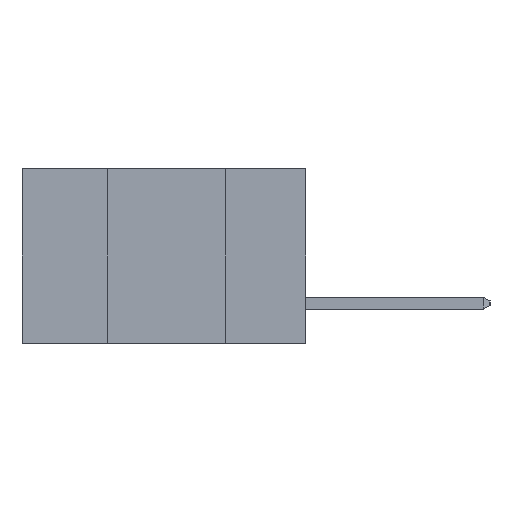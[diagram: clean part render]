
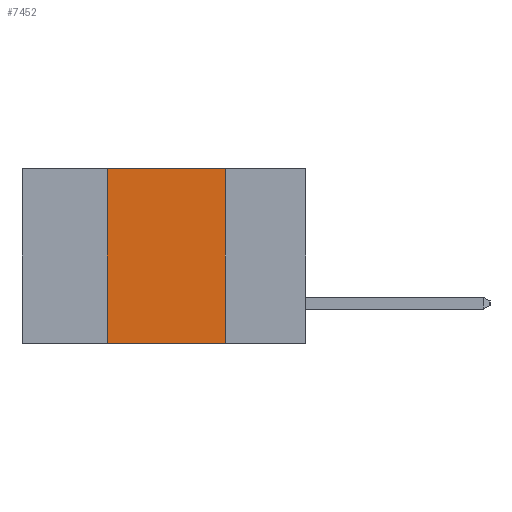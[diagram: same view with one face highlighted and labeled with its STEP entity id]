
A CAD part, left-side view. The second image highlights one B-rep face of the part: STEP entity #7452.
In plain terms, the highlighted planar face has unit normal (-1, 0, 0).
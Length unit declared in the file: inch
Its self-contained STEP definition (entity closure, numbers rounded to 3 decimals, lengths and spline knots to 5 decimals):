
#496 = DIRECTION ( 'NONE',  ( 0., 0., -1. ) ) ;
#1175 = DIRECTION ( 'NONE',  ( 0., -1., 0. ) ) ;
#1188 = DIRECTION ( 'NONE',  ( 0., 0., -1. ) ) ;
#1237 = CARTESIAN_POINT ( 'NONE',  ( 0., 0.6, -0.37 ) ) ;
#3038 = CARTESIAN_POINT ( 'NONE',  ( 0., 0.42, -0.37 ) ) ;
#3181 = ORIENTED_EDGE ( 'NONE', *, *, #9438, .F. ) ;
#3451 = CARTESIAN_POINT ( 'NONE',  ( 0., 0.6, 0. ) ) ;
#3650 = ORIENTED_EDGE ( 'NONE', *, *, #17198, .F. ) ;
#3734 = VERTEX_POINT ( 'NONE', #3038 ) ;
#5111 = FACE_OUTER_BOUND ( 'NONE', #14086, .T. ) ;
#5157 = CARTESIAN_POINT ( 'NONE',  ( 0., 0.17, 0. ) ) ;
#6205 = AXIS2_PLACEMENT_3D ( 'NONE', #3451, #9294, #496 ) ;
#6636 = ORIENTED_EDGE ( 'NONE', *, *, #11870, .F. ) ;
#6699 = EDGE_CURVE ( 'NONE', #3734, #7310, #6720, .T. ) ;
#6720 = LINE ( 'NONE', #1237, #14113 ) ;
#7310 = VERTEX_POINT ( 'NONE', #13053 ) ;
#7452 = ADVANCED_FACE ( 'NONE', ( #5111 ), #17558, .F. ) ;
#7536 = VERTEX_POINT ( 'NONE', #5157 ) ;
#9285 = CARTESIAN_POINT ( 'NONE',  ( 0., 0.42, 0. ) ) ;
#9288 = VECTOR ( 'NONE', #15101, 39.37008 ) ;
#9294 = DIRECTION ( 'NONE',  ( 1., 0., 0. ) ) ;
#9438 = EDGE_CURVE ( 'NONE', #12308, #7536, #16642, .T. ) ;
#9927 = CARTESIAN_POINT ( 'NONE',  ( 0., 0.17, 0. ) ) ;
#11161 = VECTOR ( 'NONE', #16178, 39.37008 ) ;
#11266 = ORIENTED_EDGE ( 'NONE', *, *, #6699, .T. ) ;
#11870 = EDGE_CURVE ( 'NONE', #7536, #7310, #12858, .T. ) ;
#12308 = VERTEX_POINT ( 'NONE', #17782 ) ;
#12858 = LINE ( 'NONE', #9927, #16156 ) ;
#13053 = CARTESIAN_POINT ( 'NONE',  ( 0., 0.17, -0.37 ) ) ;
#13679 = CARTESIAN_POINT ( 'NONE',  ( 0., 0.6, 0. ) ) ;
#14086 = EDGE_LOOP ( 'NONE', ( #6636, #3181, #3650, #11266 ) ) ;
#14113 = VECTOR ( 'NONE', #1175, 39.37008 ) ;
#14811 = LINE ( 'NONE', #9285, #11161 ) ;
#15101 = DIRECTION ( 'NONE',  ( 0., -1., 0. ) ) ;
#16156 = VECTOR ( 'NONE', #1188, 39.37008 ) ;
#16178 = DIRECTION ( 'NONE',  ( 0., 0., 1. ) ) ;
#16642 = LINE ( 'NONE', #13679, #9288 ) ;
#17198 = EDGE_CURVE ( 'NONE', #3734, #12308, #14811, .T. ) ;
#17558 = PLANE ( 'NONE',  #6205 ) ;
#17782 = CARTESIAN_POINT ( 'NONE',  ( 0., 0.42, 0. ) ) ;
